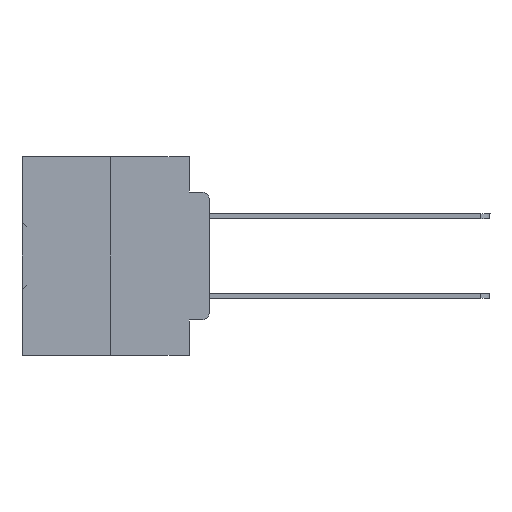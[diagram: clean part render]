
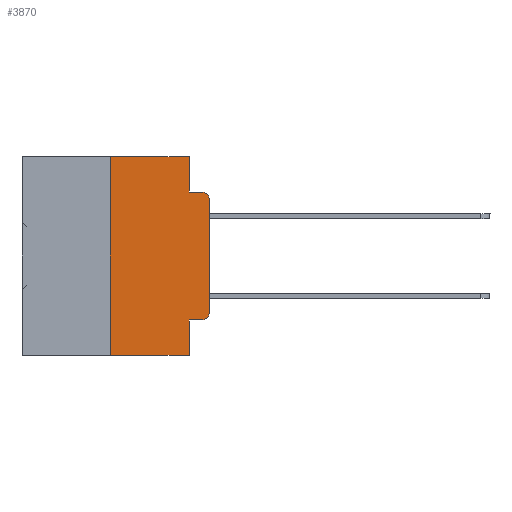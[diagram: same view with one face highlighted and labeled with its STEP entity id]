
A CAD part, left-side view. The second image highlights one B-rep face of the part: STEP entity #3870.
In plain terms, the highlighted planar face has unit normal (-1, 0, 0).
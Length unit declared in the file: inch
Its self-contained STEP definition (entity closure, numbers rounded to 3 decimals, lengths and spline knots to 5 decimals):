
#528 = VERTEX_POINT ( 'NONE', #30884 ) ;
#1106 = VECTOR ( 'NONE', #35545, 39.37008 ) ;
#1411 = EDGE_CURVE ( 'NONE', #27891, #16235, #18344, .T. ) ;
#1601 = LINE ( 'NONE', #32135, #1106 ) ;
#2086 = CIRCLE ( 'NONE', #2232, 0.02 ) ;
#2232 = AXIS2_PLACEMENT_3D ( 'NONE', #18343, #30285, #24372 ) ;
#2738 = EDGE_LOOP ( 'NONE', ( #13339, #8147, #37585, #27912, #18213, #32963, #18574, #17249, #16261, #20123 ) ) ;
#3059 = VECTOR ( 'NONE', #12798, 39.37008 ) ;
#3331 = CARTESIAN_POINT ( 'NONE',  ( 0., 0.02, -0.3915 ) ) ;
#3870 = ADVANCED_FACE ( 'NONE', ( #31095 ), #5021, .F. ) ;
#4449 = VERTEX_POINT ( 'NONE', #15585 ) ;
#5021 = PLANE ( 'NONE',  #11525 ) ;
#5226 = CARTESIAN_POINT ( 'NONE',  ( 0., 0., 0. ) ) ;
#6467 = VECTOR ( 'NONE', #24187, 39.37008 ) ;
#6725 = EDGE_CURVE ( 'NONE', #4449, #33797, #31479, .T. ) ;
#6922 = VERTEX_POINT ( 'NONE', #16587 ) ;
#7053 = LINE ( 'NONE', #25072, #32389 ) ;
#7332 = VERTEX_POINT ( 'NONE', #9721 ) ;
#7607 = EDGE_CURVE ( 'NONE', #33797, #24518, #36459, .T. ) ;
#8147 = ORIENTED_EDGE ( 'NONE', *, *, #31142, .T. ) ;
#9721 = CARTESIAN_POINT ( 'NONE',  ( 0., 0.02, -0.0885 ) ) ;
#10024 = VECTOR ( 'NONE', #20816, 39.37008 ) ;
#10272 = DIRECTION ( 'NONE',  ( 0., -1., 0. ) ) ;
#10509 = VECTOR ( 'NONE', #31115, 39.37008 ) ;
#11525 = AXIS2_PLACEMENT_3D ( 'NONE', #22774, #31520, #16473 ) ;
#11919 = CARTESIAN_POINT ( 'NONE',  ( 0., 0.051, -0.0885 ) ) ;
#12798 = DIRECTION ( 'NONE',  ( 0., 0., -1. ) ) ;
#13339 = ORIENTED_EDGE ( 'NONE', *, *, #7607, .T. ) ;
#15309 = CARTESIAN_POINT ( 'NONE',  ( 0., 0.473, 0. ) ) ;
#15585 = CARTESIAN_POINT ( 'NONE',  ( 0., 0.02, -0.4115 ) ) ;
#16235 = VERTEX_POINT ( 'NONE', #21219 ) ;
#16261 = ORIENTED_EDGE ( 'NONE', *, *, #19721, .T. ) ;
#16473 = DIRECTION ( 'NONE',  ( 0., 0., -1. ) ) ;
#16505 = VECTOR ( 'NONE', #23863, 39.37008 ) ;
#16587 = CARTESIAN_POINT ( 'NONE',  ( 0., 0.25, 0. ) ) ;
#17249 = ORIENTED_EDGE ( 'NONE', *, *, #31042, .F. ) ;
#18213 = ORIENTED_EDGE ( 'NONE', *, *, #21406, .F. ) ;
#18343 = CARTESIAN_POINT ( 'NONE',  ( 0., 0.02, -0.1085 ) ) ;
#18344 = LINE ( 'NONE', #25067, #10509 ) ;
#18441 = VERTEX_POINT ( 'NONE', #21688 ) ;
#18574 = ORIENTED_EDGE ( 'NONE', *, *, #1411, .T. ) ;
#19721 = EDGE_CURVE ( 'NONE', #18441, #4449, #7053, .T. ) ;
#20123 = ORIENTED_EDGE ( 'NONE', *, *, #6725, .T. ) ;
#20816 = DIRECTION ( 'NONE',  ( 0., -1., 0. ) ) ;
#21219 = CARTESIAN_POINT ( 'NONE',  ( 0., 0.051, -0.5 ) ) ;
#21406 = EDGE_CURVE ( 'NONE', #6922, #528, #27173, .T. ) ;
#21688 = CARTESIAN_POINT ( 'NONE',  ( 0., 0.051, -0.4115 ) ) ;
#22729 = DIRECTION ( 'NONE',  ( 0., 0., 1. ) ) ;
#22774 = CARTESIAN_POINT ( 'NONE',  ( 0., 0.473, 0. ) ) ;
#23863 = DIRECTION ( 'NONE',  ( 0., 0., 1. ) ) ;
#24187 = DIRECTION ( 'NONE',  ( 0., -1., 0. ) ) ;
#24308 = LINE ( 'NONE', #35520, #16505 ) ;
#24372 = DIRECTION ( 'NONE',  ( 0., 0., -1. ) ) ;
#24518 = VERTEX_POINT ( 'NONE', #35068 ) ;
#25067 = CARTESIAN_POINT ( 'NONE',  ( 0., 0.473, -0.5 ) ) ;
#25072 = CARTESIAN_POINT ( 'NONE',  ( 0., 0.051, -0.4115 ) ) ;
#26136 = CARTESIAN_POINT ( 'NONE',  ( 0., 0.25, -0.5 ) ) ;
#27173 = LINE ( 'NONE', #15309, #6467 ) ;
#27239 = EDGE_CURVE ( 'NONE', #27891, #6922, #24308, .T. ) ;
#27891 = VERTEX_POINT ( 'NONE', #26136 ) ;
#27912 = ORIENTED_EDGE ( 'NONE', *, *, #35614, .F. ) ;
#29114 = VECTOR ( 'NONE', #22729, 39.37008 ) ;
#29571 = DIRECTION ( 'NONE',  ( -1., 0., 0. ) ) ;
#30285 = DIRECTION ( 'NONE',  ( -1., 0., 0. ) ) ;
#30335 = CARTESIAN_POINT ( 'NONE',  ( 0., 0.051, -0.0885 ) ) ;
#30554 = CARTESIAN_POINT ( 'NONE',  ( 0., 0.051, 0. ) ) ;
#30884 = CARTESIAN_POINT ( 'NONE',  ( 0., 0.051, 0. ) ) ;
#31042 = EDGE_CURVE ( 'NONE', #18441, #16235, #1601, .T. ) ;
#31095 = FACE_OUTER_BOUND ( 'NONE', #2738, .T. ) ;
#31115 = DIRECTION ( 'NONE',  ( 0., -1., 0. ) ) ;
#31142 = EDGE_CURVE ( 'NONE', #24518, #7332, #2086, .T. ) ;
#31158 = LINE ( 'NONE', #30554, #3059 ) ;
#31479 = CIRCLE ( 'NONE', #36726, 0.02 ) ;
#31520 = DIRECTION ( 'NONE',  ( 1., 0., 0. ) ) ;
#32135 = CARTESIAN_POINT ( 'NONE',  ( 0., 0.051, 0. ) ) ;
#32389 = VECTOR ( 'NONE', #10272, 39.37008 ) ;
#32496 = VERTEX_POINT ( 'NONE', #30335 ) ;
#32548 = DIRECTION ( 'NONE',  ( 0., 0., -1. ) ) ;
#32963 = ORIENTED_EDGE ( 'NONE', *, *, #27239, .F. ) ;
#33797 = VERTEX_POINT ( 'NONE', #37222 ) ;
#35068 = CARTESIAN_POINT ( 'NONE',  ( 0., 0., -0.1085 ) ) ;
#35520 = CARTESIAN_POINT ( 'NONE',  ( 0., 0.25, 0. ) ) ;
#35545 = DIRECTION ( 'NONE',  ( 0., 0., -1. ) ) ;
#35614 = EDGE_CURVE ( 'NONE', #528, #32496, #31158, .T. ) ;
#35759 = LINE ( 'NONE', #11919, #10024 ) ;
#36459 = LINE ( 'NONE', #5226, #29114 ) ;
#36726 = AXIS2_PLACEMENT_3D ( 'NONE', #3331, #29571, #32548 ) ;
#37222 = CARTESIAN_POINT ( 'NONE',  ( 0., 0., -0.3915 ) ) ;
#37585 = ORIENTED_EDGE ( 'NONE', *, *, #37925, .F. ) ;
#37925 = EDGE_CURVE ( 'NONE', #32496, #7332, #35759, .T. ) ;
